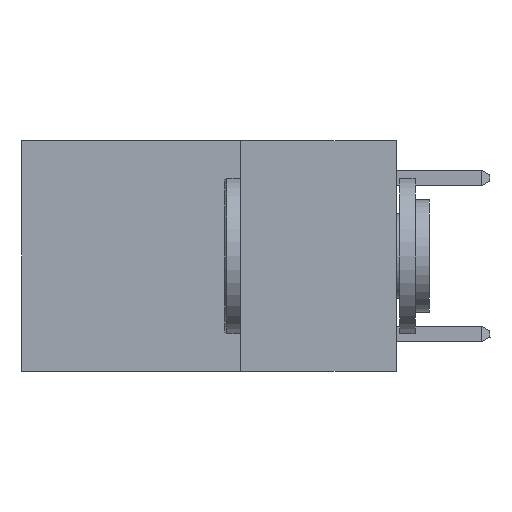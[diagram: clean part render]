
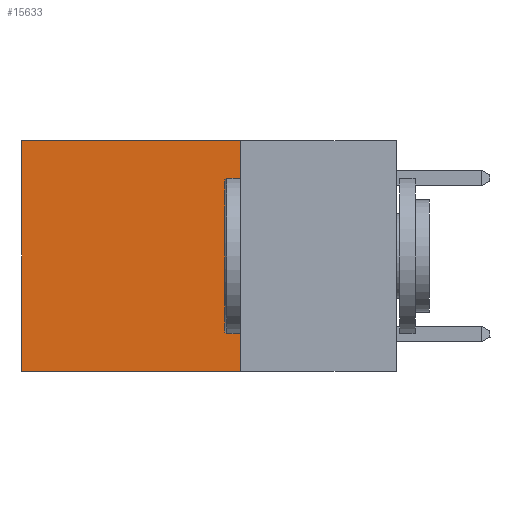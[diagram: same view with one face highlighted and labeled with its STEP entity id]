
A CAD part, left-side view. The second image highlights one B-rep face of the part: STEP entity #15633.
In plain terms, the highlighted planar face has unit normal (-1, 0, 0).
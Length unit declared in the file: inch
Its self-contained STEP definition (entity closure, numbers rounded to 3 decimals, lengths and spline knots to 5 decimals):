
#330 = CARTESIAN_POINT ( 'NONE',  ( 0.2625, 0.25, 0. ) ) ;
#478 = LINE ( 'NONE', #16905, #8500 ) ;
#678 = VECTOR ( 'NONE', #14199, 39.37008 ) ;
#731 = ORIENTED_EDGE ( 'NONE', *, *, #14907, .F. ) ;
#1517 = DIRECTION ( 'NONE',  ( 0., 1., 0. ) ) ;
#2201 = CARTESIAN_POINT ( 'NONE',  ( 0.2625, 0.6, -0.37 ) ) ;
#3737 = FACE_OUTER_BOUND ( 'NONE', #13733, .T. ) ;
#3918 = DIRECTION ( 'NONE',  ( 1., 0., 0. ) ) ;
#4702 = EDGE_CURVE ( 'NONE', #5663, #5140, #7120, .T. ) ;
#5140 = VERTEX_POINT ( 'NONE', #18572 ) ;
#5229 = DIRECTION ( 'NONE',  ( 0., 0., -1. ) ) ;
#5479 = LINE ( 'NONE', #5667, #678 ) ;
#5663 = VERTEX_POINT ( 'NONE', #13304 ) ;
#5667 = CARTESIAN_POINT ( 'NONE',  ( 0.2625, 0.25, -0.37 ) ) ;
#6118 = VERTEX_POINT ( 'NONE', #7396 ) ;
#6697 = VERTEX_POINT ( 'NONE', #2201 ) ;
#7120 = LINE ( 'NONE', #330, #13568 ) ;
#7202 = ORIENTED_EDGE ( 'NONE', *, *, #15184, .T. ) ;
#7396 = CARTESIAN_POINT ( 'NONE',  ( 0.2625, 0.6, 0. ) ) ;
#8500 = VECTOR ( 'NONE', #18134, 39.37008 ) ;
#9422 = AXIS2_PLACEMENT_3D ( 'NONE', #16789, #3918, #5229 ) ;
#10056 = DIRECTION ( 'NONE',  ( 0., 0., -1. ) ) ;
#10196 = LINE ( 'NONE', #11903, #16072 ) ;
#11092 = PLANE ( 'NONE',  #9422 ) ;
#11482 = ORIENTED_EDGE ( 'NONE', *, *, #15051, .T. ) ;
#11903 = CARTESIAN_POINT ( 'NONE',  ( 0.2625, 0.25, 0. ) ) ;
#13304 = CARTESIAN_POINT ( 'NONE',  ( 0.2625, 0.25, 0. ) ) ;
#13568 = VECTOR ( 'NONE', #10056, 39.37008 ) ;
#13733 = EDGE_LOOP ( 'NONE', ( #7202, #731, #17255, #11482 ) ) ;
#14199 = DIRECTION ( 'NONE',  ( 0., 1., 0. ) ) ;
#14907 = EDGE_CURVE ( 'NONE', #5140, #6697, #5479, .T. ) ;
#15051 = EDGE_CURVE ( 'NONE', #5663, #6118, #10196, .T. ) ;
#15184 = EDGE_CURVE ( 'NONE', #6118, #6697, #478, .T. ) ;
#15633 = ADVANCED_FACE ( 'NONE', ( #3737 ), #11092, .F. ) ;
#16072 = VECTOR ( 'NONE', #1517, 39.37008 ) ;
#16789 = CARTESIAN_POINT ( 'NONE',  ( 0.2625, 0.25, 0. ) ) ;
#16905 = CARTESIAN_POINT ( 'NONE',  ( 0.2625, 0.6, 0. ) ) ;
#17255 = ORIENTED_EDGE ( 'NONE', *, *, #4702, .F. ) ;
#18134 = DIRECTION ( 'NONE',  ( 0., 0., -1. ) ) ;
#18572 = CARTESIAN_POINT ( 'NONE',  ( 0.2625, 0.25, -0.37 ) ) ;
